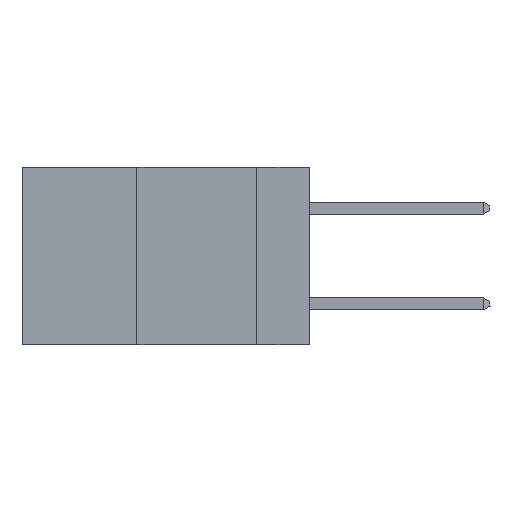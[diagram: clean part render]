
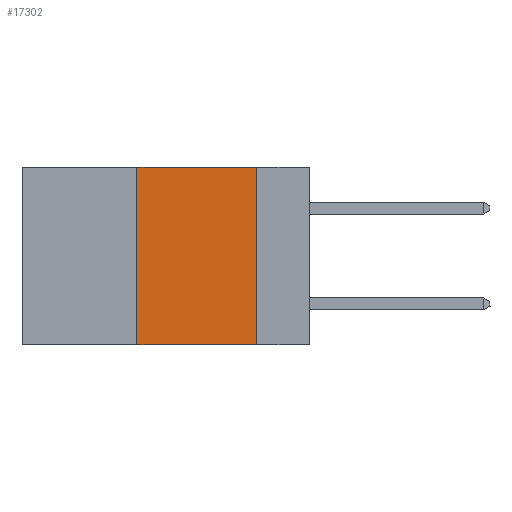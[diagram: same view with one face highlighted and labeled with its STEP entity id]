
A CAD part, left-side view. The second image highlights one B-rep face of the part: STEP entity #17302.
In plain terms, the highlighted planar face has unit normal (-1, 0, 0).
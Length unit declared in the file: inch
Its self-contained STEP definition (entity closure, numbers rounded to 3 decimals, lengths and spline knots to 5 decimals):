
#403 = EDGE_CURVE ( 'NONE', #7611, #27596, #19307, .T. ) ;
#505 = VECTOR ( 'NONE', #17262, 39.37008 ) ;
#3790 = ORIENTED_EDGE ( 'NONE', *, *, #11724, .T. ) ;
#5028 = PLANE ( 'NONE',  #14918 ) ;
#5127 = DIRECTION ( 'NONE',  ( 0., 0., -1. ) ) ;
#5721 = CARTESIAN_POINT ( 'NONE',  ( 0., 0.36, 0. ) ) ;
#6345 = LINE ( 'NONE', #22757, #11970 ) ;
#6599 = VECTOR ( 'NONE', #10909, 39.37008 ) ;
#7611 = VERTEX_POINT ( 'NONE', #11232 ) ;
#9061 = ORIENTED_EDGE ( 'NONE', *, *, #403, .F. ) ;
#10514 = CARTESIAN_POINT ( 'NONE',  ( 0., 0.6, 0. ) ) ;
#10909 = DIRECTION ( 'NONE',  ( 0., -1., 0. ) ) ;
#11232 = CARTESIAN_POINT ( 'NONE',  ( 0., 0.36, 0. ) ) ;
#11724 = EDGE_CURVE ( 'NONE', #19629, #27192, #25627, .T. ) ;
#11970 = VECTOR ( 'NONE', #16359, 39.37008 ) ;
#11979 = EDGE_CURVE ( 'NONE', #19629, #7611, #20979, .T. ) ;
#12062 = ORIENTED_EDGE ( 'NONE', *, *, #11979, .F. ) ;
#12117 = CARTESIAN_POINT ( 'NONE',  ( 0., 0.11, -0.37 ) ) ;
#14918 = AXIS2_PLACEMENT_3D ( 'NONE', #22846, #20786, #5127 ) ;
#15062 = CARTESIAN_POINT ( 'NONE',  ( 0., 0.36, -0.37 ) ) ;
#16359 = DIRECTION ( 'NONE',  ( 0., 0., -1. ) ) ;
#16567 = FACE_OUTER_BOUND ( 'NONE', #27684, .T. ) ;
#17262 = DIRECTION ( 'NONE',  ( 0., 0., 1. ) ) ;
#17302 = ADVANCED_FACE ( 'NONE', ( #16567 ), #5028, .F. ) ;
#19307 = LINE ( 'NONE', #10514, #6599 ) ;
#19629 = VERTEX_POINT ( 'NONE', #15062 ) ;
#20390 = CARTESIAN_POINT ( 'NONE',  ( 0., 0.6, -0.37 ) ) ;
#20786 = DIRECTION ( 'NONE',  ( 1., 0., 0. ) ) ;
#20979 = LINE ( 'NONE', #5721, #505 ) ;
#21155 = DIRECTION ( 'NONE',  ( 0., -1., 0. ) ) ;
#22757 = CARTESIAN_POINT ( 'NONE',  ( 0., 0.11, 0. ) ) ;
#22846 = CARTESIAN_POINT ( 'NONE',  ( 0., 0.6, 0. ) ) ;
#23295 = EDGE_CURVE ( 'NONE', #27596, #27192, #6345, .T. ) ;
#25627 = LINE ( 'NONE', #20390, #28836 ) ;
#26493 = ORIENTED_EDGE ( 'NONE', *, *, #23295, .F. ) ;
#27192 = VERTEX_POINT ( 'NONE', #12117 ) ;
#27524 = CARTESIAN_POINT ( 'NONE',  ( 0., 0.11, 0. ) ) ;
#27596 = VERTEX_POINT ( 'NONE', #27524 ) ;
#27684 = EDGE_LOOP ( 'NONE', ( #26493, #9061, #12062, #3790 ) ) ;
#28836 = VECTOR ( 'NONE', #21155, 39.37008 ) ;
